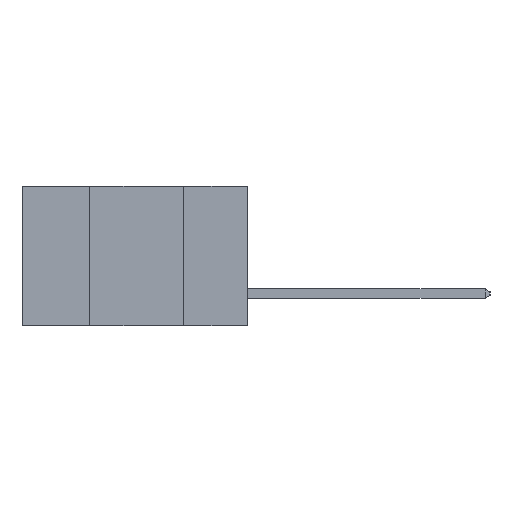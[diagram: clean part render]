
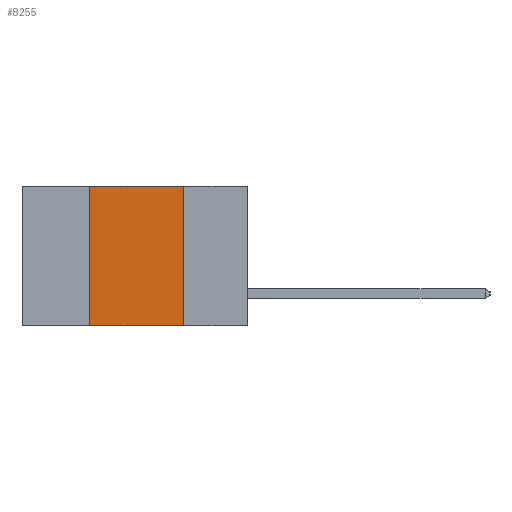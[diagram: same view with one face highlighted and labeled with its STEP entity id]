
A CAD part, left-side view. The second image highlights one B-rep face of the part: STEP entity #8255.
In plain terms, the highlighted planar face has unit normal (-1, 0, 0).
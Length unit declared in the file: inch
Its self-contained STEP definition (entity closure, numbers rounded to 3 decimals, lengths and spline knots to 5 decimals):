
#47 = CARTESIAN_POINT ( 'NONE',  ( 0., 0.42, 0. ) ) ;
#141 = ORIENTED_EDGE ( 'NONE', *, *, #4171, .F. ) ;
#906 = VECTOR ( 'NONE', #8351, 39.37008 ) ;
#1917 = VERTEX_POINT ( 'NONE', #4670 ) ;
#2053 = LINE ( 'NONE', #3670, #5383 ) ;
#2195 = ORIENTED_EDGE ( 'NONE', *, *, #4907, .T. ) ;
#3454 = CARTESIAN_POINT ( 'NONE',  ( 0., 0.17, -0.37 ) ) ;
#3526 = VECTOR ( 'NONE', #7066, 39.37008 ) ;
#3670 = CARTESIAN_POINT ( 'NONE',  ( 0., 0.42, -0.37 ) ) ;
#3859 = VERTEX_POINT ( 'NONE', #5905 ) ;
#4126 = DIRECTION ( 'NONE',  ( 0., 0., 1. ) ) ;
#4158 = DIRECTION ( 'NONE',  ( 0., 0., -1. ) ) ;
#4171 = EDGE_CURVE ( 'NONE', #1917, #6493, #2053, .T. ) ;
#4468 = EDGE_LOOP ( 'NONE', ( #4824, #6507, #141, #2195 ) ) ;
#4670 = CARTESIAN_POINT ( 'NONE',  ( 0., 0.42, -0.37 ) ) ;
#4824 = ORIENTED_EDGE ( 'NONE', *, *, #7555, .F. ) ;
#4907 = EDGE_CURVE ( 'NONE', #1917, #7673, #8397, .T. ) ;
#5383 = VECTOR ( 'NONE', #4126, 39.37008 ) ;
#5452 = PLANE ( 'NONE',  #8367 ) ;
#5549 = CARTESIAN_POINT ( 'NONE',  ( 0., 0.17, -0.37 ) ) ;
#5736 = LINE ( 'NONE', #7759, #7346 ) ;
#5905 = CARTESIAN_POINT ( 'NONE',  ( 0., 0.17, 0. ) ) ;
#5963 = DIRECTION ( 'NONE',  ( 0., -1., 0. ) ) ;
#6065 = CARTESIAN_POINT ( 'NONE',  ( 0., 0.6, 0. ) ) ;
#6099 = LINE ( 'NONE', #3454, #906 ) ;
#6493 = VERTEX_POINT ( 'NONE', #47 ) ;
#6507 = ORIENTED_EDGE ( 'NONE', *, *, #6771, .F. ) ;
#6771 = EDGE_CURVE ( 'NONE', #6493, #3859, #5736, .T. ) ;
#6856 = FACE_OUTER_BOUND ( 'NONE', #4468, .T. ) ;
#7066 = DIRECTION ( 'NONE',  ( 0., -1., 0. ) ) ;
#7273 = CARTESIAN_POINT ( 'NONE',  ( 0., 0.6, -0.37 ) ) ;
#7346 = VECTOR ( 'NONE', #5963, 39.37008 ) ;
#7555 = EDGE_CURVE ( 'NONE', #3859, #7673, #6099, .T. ) ;
#7673 = VERTEX_POINT ( 'NONE', #5549 ) ;
#7759 = CARTESIAN_POINT ( 'NONE',  ( 0., 0.6, 0. ) ) ;
#7843 = DIRECTION ( 'NONE',  ( 1., 0., 0. ) ) ;
#8255 = ADVANCED_FACE ( 'NONE', ( #6856 ), #5452, .F. ) ;
#8351 = DIRECTION ( 'NONE',  ( 0., 0., -1. ) ) ;
#8367 = AXIS2_PLACEMENT_3D ( 'NONE', #6065, #7843, #4158 ) ;
#8397 = LINE ( 'NONE', #7273, #3526 ) ;
